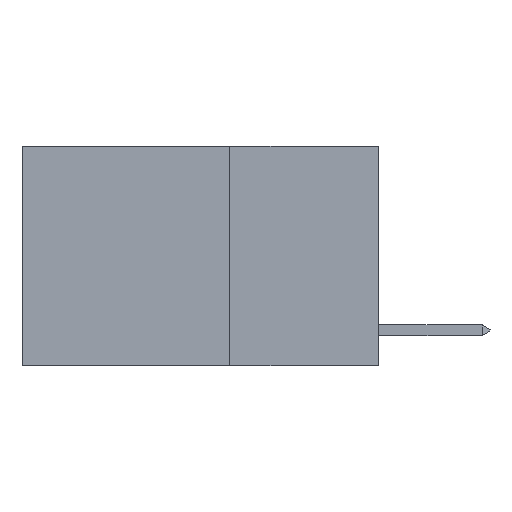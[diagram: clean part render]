
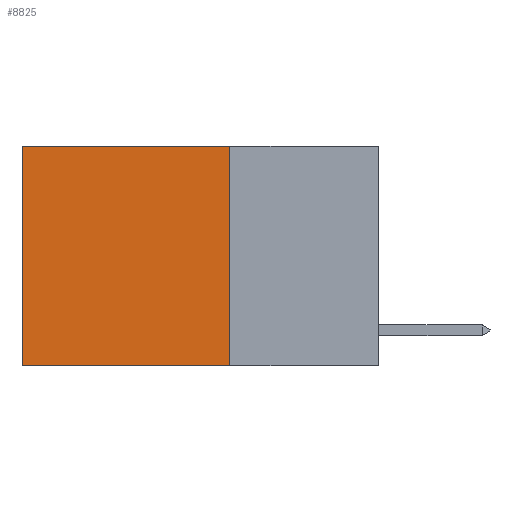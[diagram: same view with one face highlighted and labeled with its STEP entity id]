
A CAD part, left-side view. The second image highlights one B-rep face of the part: STEP entity #8825.
In plain terms, the highlighted planar face has unit normal (-1, 0, 0).
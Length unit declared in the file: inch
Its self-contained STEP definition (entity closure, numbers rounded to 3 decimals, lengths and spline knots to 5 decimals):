
#128 = EDGE_CURVE ( 'NONE', #9964, #12776, #13925, .T. ) ;
#929 = CARTESIAN_POINT ( 'NONE',  ( 0.2625, 0.6, -0.37 ) ) ;
#967 = VECTOR ( 'NONE', #6498, 39.37008 ) ;
#990 = VECTOR ( 'NONE', #11659, 39.37008 ) ;
#1497 = VERTEX_POINT ( 'NONE', #4486 ) ;
#4486 = CARTESIAN_POINT ( 'NONE',  ( 0.2625, 0.25, 0. ) ) ;
#4657 = VECTOR ( 'NONE', #7233, 39.37008 ) ;
#4903 = ORIENTED_EDGE ( 'NONE', *, *, #5297, .F. ) ;
#5018 = EDGE_CURVE ( 'NONE', #1497, #9617, #14314, .T. ) ;
#5248 = DIRECTION ( 'NONE',  ( 1., 0., 0. ) ) ;
#5297 = EDGE_CURVE ( 'NONE', #1497, #9964, #8848, .T. ) ;
#6096 = ORIENTED_EDGE ( 'NONE', *, *, #5018, .T. ) ;
#6407 = EDGE_CURVE ( 'NONE', #9617, #12776, #7081, .T. ) ;
#6498 = DIRECTION ( 'NONE',  ( 0., 0., -1. ) ) ;
#6733 = ORIENTED_EDGE ( 'NONE', *, *, #128, .F. ) ;
#6857 = DIRECTION ( 'NONE',  ( 0., 0., -1. ) ) ;
#7081 = LINE ( 'NONE', #14946, #967 ) ;
#7233 = DIRECTION ( 'NONE',  ( 0., 1., 0. ) ) ;
#7407 = CARTESIAN_POINT ( 'NONE',  ( 0.2625, 0.25, -0.37 ) ) ;
#8018 = ORIENTED_EDGE ( 'NONE', *, *, #6407, .T. ) ;
#8825 = ADVANCED_FACE ( 'NONE', ( #9136 ), #12482, .F. ) ;
#8848 = LINE ( 'NONE', #9269, #10562 ) ;
#9136 = FACE_OUTER_BOUND ( 'NONE', #12619, .T. ) ;
#9269 = CARTESIAN_POINT ( 'NONE',  ( 0.2625, 0.25, 0. ) ) ;
#9617 = VERTEX_POINT ( 'NONE', #12889 ) ;
#9964 = VERTEX_POINT ( 'NONE', #7407 ) ;
#10098 = CARTESIAN_POINT ( 'NONE',  ( 0.2625, 0.25, 0. ) ) ;
#10434 = CARTESIAN_POINT ( 'NONE',  ( 0.2625, 0.25, -0.37 ) ) ;
#10562 = VECTOR ( 'NONE', #6857, 39.37008 ) ;
#11659 = DIRECTION ( 'NONE',  ( 0., 1., 0. ) ) ;
#12482 = PLANE ( 'NONE',  #14358 ) ;
#12619 = EDGE_LOOP ( 'NONE', ( #8018, #6733, #4903, #6096 ) ) ;
#12776 = VERTEX_POINT ( 'NONE', #929 ) ;
#12889 = CARTESIAN_POINT ( 'NONE',  ( 0.2625, 0.6, 0. ) ) ;
#13278 = CARTESIAN_POINT ( 'NONE',  ( 0.2625, 0.25, 0. ) ) ;
#13739 = DIRECTION ( 'NONE',  ( 0., 0., -1. ) ) ;
#13925 = LINE ( 'NONE', #10434, #990 ) ;
#14314 = LINE ( 'NONE', #13278, #4657 ) ;
#14358 = AXIS2_PLACEMENT_3D ( 'NONE', #10098, #5248, #13739 ) ;
#14946 = CARTESIAN_POINT ( 'NONE',  ( 0.2625, 0.6, 0. ) ) ;
